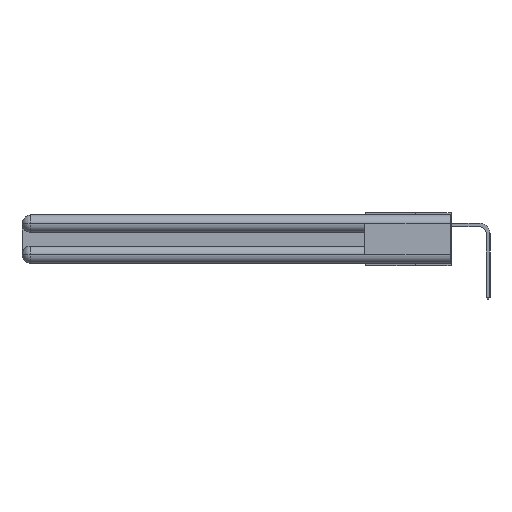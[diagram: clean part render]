
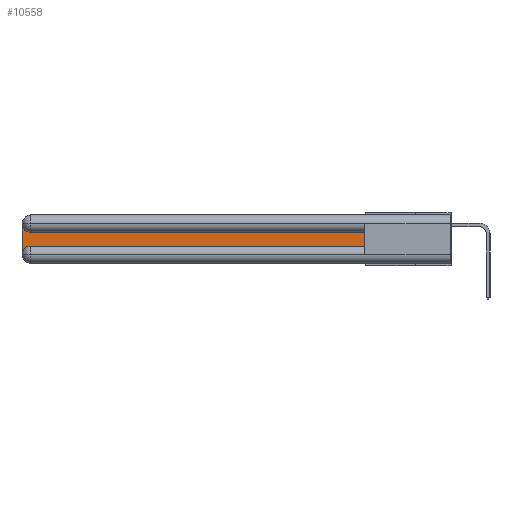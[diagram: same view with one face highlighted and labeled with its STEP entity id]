
A CAD part, left-side view. The second image highlights one B-rep face of the part: STEP entity #10558.
In plain terms, the highlighted planar face has unit normal (-1, 0, 0).
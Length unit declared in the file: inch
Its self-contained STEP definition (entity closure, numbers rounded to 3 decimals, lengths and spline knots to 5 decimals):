
#482 = DIRECTION ( 'NONE',  ( 1., 0., 0. ) ) ;
#1166 = EDGE_CURVE ( 'NONE', #12416, #25076, #14040, .T. ) ;
#1742 = DIRECTION ( 'NONE',  ( 0., 0., -1. ) ) ;
#1941 = PLANE ( 'NONE',  #28083 ) ;
#2683 = EDGE_CURVE ( 'NONE', #7978, #20442, #9207, .T. ) ;
#2688 = VECTOR ( 'NONE', #3508, 39.37008 ) ;
#3069 = ORIENTED_EDGE ( 'NONE', *, *, #1166, .T. ) ;
#3508 = DIRECTION ( 'NONE',  ( 0., 1., 0. ) ) ;
#3997 = CARTESIAN_POINT ( 'NONE',  ( 0.075, 3., -0.2175 ) ) ;
#7541 = ORIENTED_EDGE ( 'NONE', *, *, #21410, .T. ) ;
#7542 = VERTEX_POINT ( 'NONE', #14965 ) ;
#7559 = ORIENTED_EDGE ( 'NONE', *, *, #9059, .T. ) ;
#7978 = VERTEX_POINT ( 'NONE', #25769 ) ;
#8805 = CIRCLE ( 'NONE', #25138, 0.06 ) ;
#8906 = DIRECTION ( 'NONE',  ( 0., 0., -1. ) ) ;
#9059 = EDGE_CURVE ( 'NONE', #20442, #12416, #16254, .T. ) ;
#9207 = LINE ( 'NONE', #12934, #21284 ) ;
#9510 = DIRECTION ( 'NONE',  ( 0., 0., -1. ) ) ;
#9686 = CARTESIAN_POINT ( 'NONE',  ( 0.075, 0.6, -0.2175 ) ) ;
#9847 = LINE ( 'NONE', #3997, #23739 ) ;
#9882 = CIRCLE ( 'NONE', #28622, 0.06 ) ;
#10558 = ADVANCED_FACE ( 'NONE', ( #12149 ), #1941, .F. ) ;
#11512 = EDGE_LOOP ( 'NONE', ( #3069, #7541, #28069, #19902, #27589, #7559 ) ) ;
#12149 = FACE_OUTER_BOUND ( 'NONE', #11512, .T. ) ;
#12416 = VERTEX_POINT ( 'NONE', #26745 ) ;
#12934 = CARTESIAN_POINT ( 'NONE',  ( 0.075, 0.6, -0.2175 ) ) ;
#13489 = DIRECTION ( 'NONE',  ( 1., 0., 0. ) ) ;
#13943 = DIRECTION ( 'NONE',  ( 1., 0., 0. ) ) ;
#14040 = LINE ( 'NONE', #15072, #2688 ) ;
#14965 = CARTESIAN_POINT ( 'NONE',  ( 0.075, 3., -0.0625 ) ) ;
#15072 = CARTESIAN_POINT ( 'NONE',  ( 0.075, 0.6, -0.1225 ) ) ;
#15257 = DIRECTION ( 'NONE',  ( 0., -1., 0. ) ) ;
#15829 = DIRECTION ( 'NONE',  ( 0., 0., -1. ) ) ;
#16254 = LINE ( 'NONE', #19148, #21029 ) ;
#17706 = CARTESIAN_POINT ( 'NONE',  ( 0.075, 2.94, -0.1225 ) ) ;
#18063 = CARTESIAN_POINT ( 'NONE',  ( 0.075, 2.94, -0.2775 ) ) ;
#18537 = EDGE_CURVE ( 'NONE', #27158, #7978, #9882, .T. ) ;
#19148 = CARTESIAN_POINT ( 'NONE',  ( 0.075, 0.6, -0.2175 ) ) ;
#19902 = ORIENTED_EDGE ( 'NONE', *, *, #18537, .T. ) ;
#20442 = VERTEX_POINT ( 'NONE', #9686 ) ;
#20893 = CARTESIAN_POINT ( 'NONE',  ( 0.075, 3., -0.1225 ) ) ;
#21029 = VECTOR ( 'NONE', #25974, 39.37008 ) ;
#21284 = VECTOR ( 'NONE', #15257, 39.37008 ) ;
#21410 = EDGE_CURVE ( 'NONE', #25076, #7542, #8805, .T. ) ;
#21484 = CARTESIAN_POINT ( 'NONE',  ( 0.075, 2.94, -0.0625 ) ) ;
#23739 = VECTOR ( 'NONE', #1742, 39.37008 ) ;
#25076 = VERTEX_POINT ( 'NONE', #17706 ) ;
#25138 = AXIS2_PLACEMENT_3D ( 'NONE', #21484, #482, #9510 ) ;
#25769 = CARTESIAN_POINT ( 'NONE',  ( 0.075, 2.94, -0.2175 ) ) ;
#25974 = DIRECTION ( 'NONE',  ( 0., 0., 1. ) ) ;
#26745 = CARTESIAN_POINT ( 'NONE',  ( 0.075, 0.6, -0.1225 ) ) ;
#27158 = VERTEX_POINT ( 'NONE', #29914 ) ;
#27589 = ORIENTED_EDGE ( 'NONE', *, *, #2683, .T. ) ;
#28069 = ORIENTED_EDGE ( 'NONE', *, *, #29011, .T. ) ;
#28083 = AXIS2_PLACEMENT_3D ( 'NONE', #20893, #13943, #8906 ) ;
#28622 = AXIS2_PLACEMENT_3D ( 'NONE', #18063, #13489, #15829 ) ;
#29011 = EDGE_CURVE ( 'NONE', #7542, #27158, #9847, .T. ) ;
#29914 = CARTESIAN_POINT ( 'NONE',  ( 0.075, 3., -0.2775 ) ) ;
